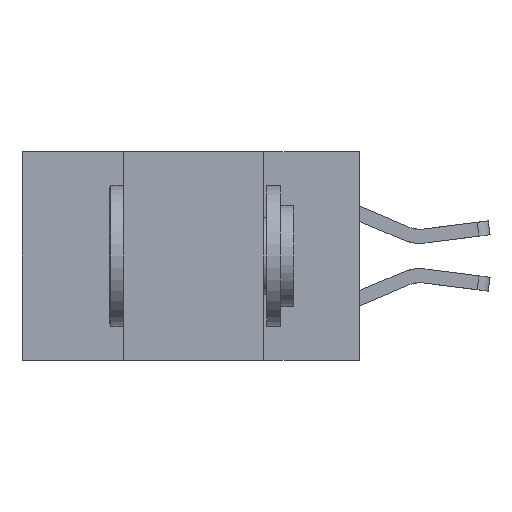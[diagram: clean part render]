
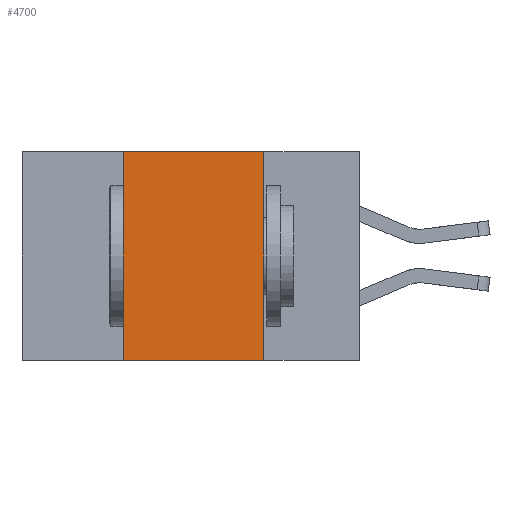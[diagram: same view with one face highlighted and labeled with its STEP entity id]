
A CAD part, left-side view. The second image highlights one B-rep face of the part: STEP entity #4700.
In plain terms, the highlighted planar face has unit normal (-1, 0, 0).
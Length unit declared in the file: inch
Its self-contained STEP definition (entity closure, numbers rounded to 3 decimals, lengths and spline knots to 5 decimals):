
#160 = AXIS2_PLACEMENT_3D ( 'NONE', #11090, #4903, #12296 ) ;
#808 = ORIENTED_EDGE ( 'NONE', *, *, #8163, .F. ) ;
#1501 = DIRECTION ( 'NONE',  ( 0., -1., 0. ) ) ;
#2064 = EDGE_LOOP ( 'NONE', ( #11785, #9434, #808, #2665 ) ) ;
#2248 = LINE ( 'NONE', #4332, #4114 ) ;
#2506 = LINE ( 'NONE', #5440, #3037 ) ;
#2635 = LINE ( 'NONE', #5596, #6669 ) ;
#2665 = ORIENTED_EDGE ( 'NONE', *, *, #11247, .T. ) ;
#3037 = VECTOR ( 'NONE', #12948, 39.37008 ) ;
#3630 = VERTEX_POINT ( 'NONE', #5879 ) ;
#4114 = VECTOR ( 'NONE', #4147, 39.37008 ) ;
#4147 = DIRECTION ( 'NONE',  ( 0., -1., 0. ) ) ;
#4332 = CARTESIAN_POINT ( 'NONE',  ( 0., 0.6, -0.37 ) ) ;
#4403 = CARTESIAN_POINT ( 'NONE',  ( 0., 0.42, 0. ) ) ;
#4700 = ADVANCED_FACE ( 'NONE', ( #13167 ), #12158, .F. ) ;
#4903 = DIRECTION ( 'NONE',  ( 1., 0., 0. ) ) ;
#5384 = LINE ( 'NONE', #11954, #13441 ) ;
#5440 = CARTESIAN_POINT ( 'NONE',  ( 0., 0.42, 0. ) ) ;
#5596 = CARTESIAN_POINT ( 'NONE',  ( 0., 0.6, 0. ) ) ;
#5603 = VERTEX_POINT ( 'NONE', #8306 ) ;
#5879 = CARTESIAN_POINT ( 'NONE',  ( 0., 0.17, -0.37 ) ) ;
#6669 = VECTOR ( 'NONE', #1501, 39.37008 ) ;
#7158 = EDGE_CURVE ( 'NONE', #5603, #3630, #5384, .T. ) ;
#7832 = CARTESIAN_POINT ( 'NONE',  ( 0., 0.42, -0.37 ) ) ;
#8163 = EDGE_CURVE ( 'NONE', #12909, #11021, #2506, .T. ) ;
#8306 = CARTESIAN_POINT ( 'NONE',  ( 0., 0.17, 0. ) ) ;
#9196 = EDGE_CURVE ( 'NONE', #11021, #5603, #2635, .T. ) ;
#9434 = ORIENTED_EDGE ( 'NONE', *, *, #9196, .F. ) ;
#11021 = VERTEX_POINT ( 'NONE', #4403 ) ;
#11090 = CARTESIAN_POINT ( 'NONE',  ( 0., 0.6, 0. ) ) ;
#11247 = EDGE_CURVE ( 'NONE', #12909, #3630, #2248, .T. ) ;
#11785 = ORIENTED_EDGE ( 'NONE', *, *, #7158, .F. ) ;
#11954 = CARTESIAN_POINT ( 'NONE',  ( 0., 0.17, 0. ) ) ;
#12158 = PLANE ( 'NONE',  #160 ) ;
#12296 = DIRECTION ( 'NONE',  ( 0., 0., -1. ) ) ;
#12909 = VERTEX_POINT ( 'NONE', #7832 ) ;
#12948 = DIRECTION ( 'NONE',  ( 0., 0., 1. ) ) ;
#12986 = DIRECTION ( 'NONE',  ( 0., 0., -1. ) ) ;
#13167 = FACE_OUTER_BOUND ( 'NONE', #2064, .T. ) ;
#13441 = VECTOR ( 'NONE', #12986, 39.37008 ) ;
